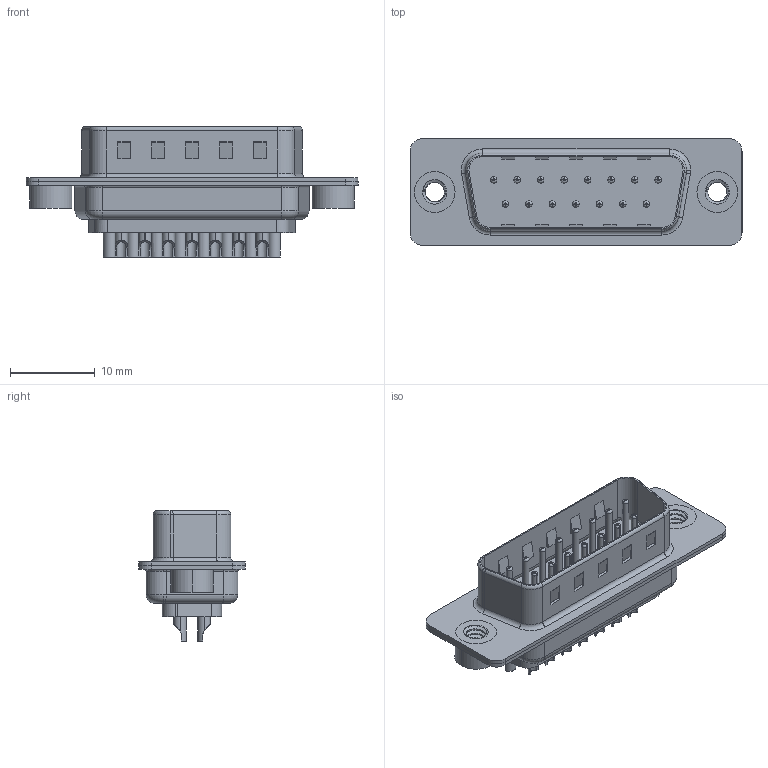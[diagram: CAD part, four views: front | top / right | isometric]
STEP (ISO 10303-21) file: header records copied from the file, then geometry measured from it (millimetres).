
FILE_DESCRIPTION (( 'STEP AP203' ), '1' );
FILE_NAME ('627-015-322-542.STEP', '2018-10-04T04:58:40', ( '' ), ( '' ), 'SwSTEP 2.0', 'SolidWorks 2016', '' );
FILE_SCHEMA (( 'CONFIG_CONTROL_DESIGN' ));
Length unit declared in the file: millimetre
Products named in the file (7): 627 Shell Front_15 Contacts; 627 Shell Rear_15 Contacts; 627 Contact Row 1_22L; 627 Contact Row 2_22L; 627 4-40 Threaded Rivet; 627-015-322-542; 627 Housing_15 LP
Assembly tree (20 placements, depth 2):
  627-015-322-542
    627 Housing_15 LP
    627 Shell Front_15 Contacts
    627 Shell Rear_15 Contacts
    627 Contact Row 1_22L  x8
    627 Contact Row 2_22L  x7
    627 4-40 Threaded Rivet  x2
Bounding box: 39.15 x 12.6 x 15.35 mm (x, y, z)
Volume: 1838.1 mm3; surface area: 5429.6 mm2
Topology: 20 solids, 20 shells, 1300 faces, 3319 edges, 2100 vertices
Faces by surface type: cylinder 568, torus 371, plane 349, cone 6, bspline 6
Entity records: 18908 total; most frequent: CARTESIAN_POINT 4406, DIRECTION 3015, ORIENTED_EDGE 2678, EDGE_CURVE 1339, AXIS2_PLACEMENT_3D 1190, VERTEX_POINT 851, EDGE_LOOP 642, VECTOR 635
